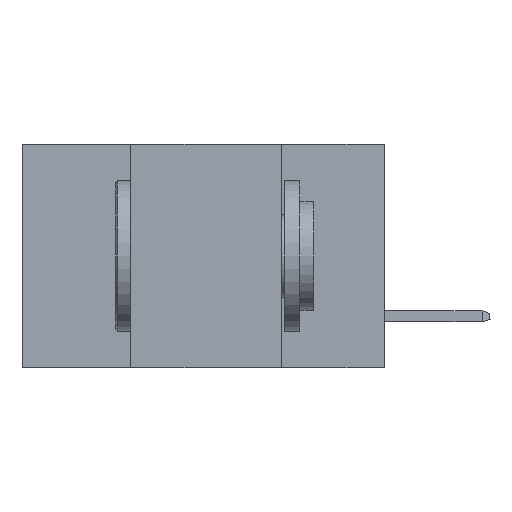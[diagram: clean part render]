
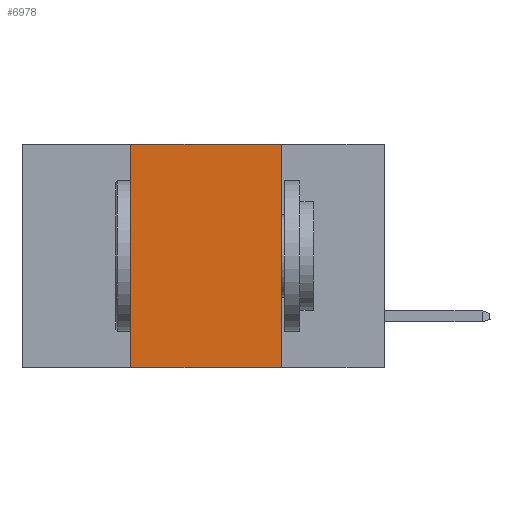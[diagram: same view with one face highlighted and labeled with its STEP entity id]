
A CAD part, left-side view. The second image highlights one B-rep face of the part: STEP entity #6978.
In plain terms, the highlighted planar face has unit normal (-1, 0, 0).
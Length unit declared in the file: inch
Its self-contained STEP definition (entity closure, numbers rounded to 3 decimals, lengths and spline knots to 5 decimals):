
#613 = ORIENTED_EDGE ( 'NONE', *, *, #6126, .F. ) ;
#830 = DIRECTION ( 'NONE',  ( 0., 0., -1. ) ) ;
#946 = ORIENTED_EDGE ( 'NONE', *, *, #3063, .F. ) ;
#1049 = LINE ( 'NONE', #11360, #10919 ) ;
#1236 = AXIS2_PLACEMENT_3D ( 'NONE', #5315, #9170, #4423 ) ;
#2069 = ORIENTED_EDGE ( 'NONE', *, *, #7424, .T. ) ;
#2723 = FACE_OUTER_BOUND ( 'NONE', #3925, .T. ) ;
#2825 = CARTESIAN_POINT ( 'NONE',  ( 0., 0.17, 0. ) ) ;
#3063 = EDGE_CURVE ( 'NONE', #7625, #3555, #1049, .T. ) ;
#3362 = DIRECTION ( 'NONE',  ( 0., -1., 0. ) ) ;
#3555 = VERTEX_POINT ( 'NONE', #11372 ) ;
#3907 = VECTOR ( 'NONE', #3362, 39.37008 ) ;
#3925 = EDGE_LOOP ( 'NONE', ( #613, #11280, #946, #2069 ) ) ;
#4213 = CARTESIAN_POINT ( 'NONE',  ( 0., 0.6, 0. ) ) ;
#4423 = DIRECTION ( 'NONE',  ( 0., 0., -1. ) ) ;
#5315 = CARTESIAN_POINT ( 'NONE',  ( 0., 0.6, 0. ) ) ;
#5397 = PLANE ( 'NONE',  #1236 ) ;
#5591 = VECTOR ( 'NONE', #6592, 39.37008 ) ;
#5877 = CARTESIAN_POINT ( 'NONE',  ( 0., 0.17, -0.37 ) ) ;
#5995 = CARTESIAN_POINT ( 'NONE',  ( 0., 0.42, -0.37 ) ) ;
#6054 = VECTOR ( 'NONE', #830, 39.37008 ) ;
#6126 = EDGE_CURVE ( 'NONE', #11988, #6308, #10823, .T. ) ;
#6308 = VERTEX_POINT ( 'NONE', #5877 ) ;
#6592 = DIRECTION ( 'NONE',  ( 0., -1., 0. ) ) ;
#6978 = ADVANCED_FACE ( 'NONE', ( #2723 ), #5397, .F. ) ;
#7424 = EDGE_CURVE ( 'NONE', #7625, #6308, #8691, .T. ) ;
#7625 = VERTEX_POINT ( 'NONE', #5995 ) ;
#8691 = LINE ( 'NONE', #11352, #5591 ) ;
#8701 = EDGE_CURVE ( 'NONE', #3555, #11988, #10921, .T. ) ;
#9170 = DIRECTION ( 'NONE',  ( 1., 0., 0. ) ) ;
#9321 = CARTESIAN_POINT ( 'NONE',  ( 0., 0.17, 0. ) ) ;
#10251 = DIRECTION ( 'NONE',  ( 0., 0., 1. ) ) ;
#10823 = LINE ( 'NONE', #9321, #6054 ) ;
#10919 = VECTOR ( 'NONE', #10251, 39.37008 ) ;
#10921 = LINE ( 'NONE', #4213, #3907 ) ;
#11280 = ORIENTED_EDGE ( 'NONE', *, *, #8701, .F. ) ;
#11352 = CARTESIAN_POINT ( 'NONE',  ( 0., 0.6, -0.37 ) ) ;
#11360 = CARTESIAN_POINT ( 'NONE',  ( 0., 0.42, 0. ) ) ;
#11372 = CARTESIAN_POINT ( 'NONE',  ( 0., 0.42, 0. ) ) ;
#11988 = VERTEX_POINT ( 'NONE', #2825 ) ;
